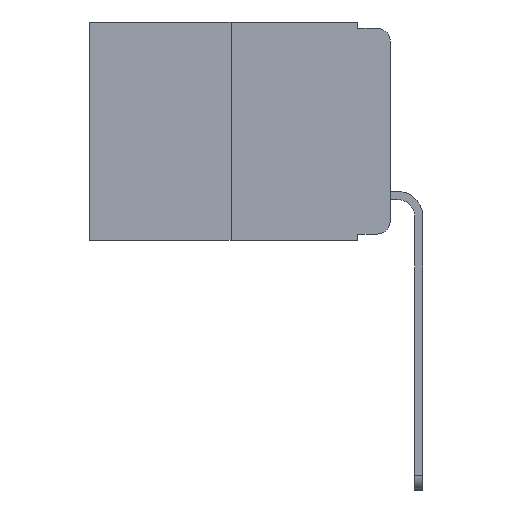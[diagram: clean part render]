
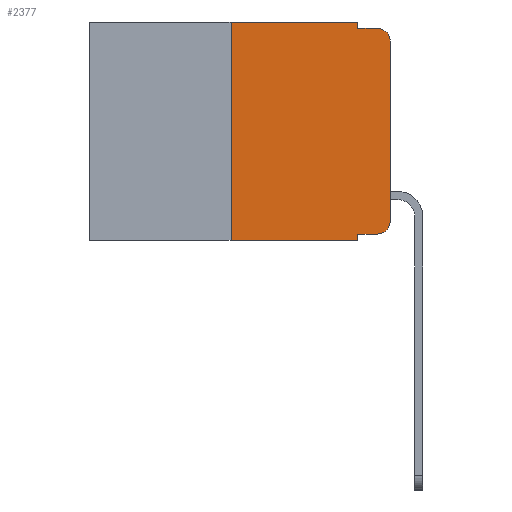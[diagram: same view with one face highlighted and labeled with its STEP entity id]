
A CAD part, left-side view. The second image highlights one B-rep face of the part: STEP entity #2377.
In plain terms, the highlighted planar face has unit normal (-1, 0, 0).
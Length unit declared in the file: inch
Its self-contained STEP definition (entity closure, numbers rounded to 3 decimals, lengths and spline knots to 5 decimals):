
#36 = VERTEX_POINT ( 'NONE', #1547 ) ;
#52 = DIRECTION ( 'NONE',  ( 0., 0., -1. ) ) ;
#395 = CARTESIAN_POINT ( 'NONE',  ( 0., 0.25, -0.343 ) ) ;
#418 = CARTESIAN_POINT ( 'NONE',  ( 0., 0.473, 0. ) ) ;
#467 = DIRECTION ( 'NONE',  ( 0., -1., 0. ) ) ;
#686 = EDGE_CURVE ( 'NONE', #36, #824, #2231, .T. ) ;
#691 = CARTESIAN_POINT ( 'NONE',  ( 0., 0.051, 0. ) ) ;
#729 = DIRECTION ( 'NONE',  ( 0., 0., -1. ) ) ;
#824 = VERTEX_POINT ( 'NONE', #7300 ) ;
#953 = VERTEX_POINT ( 'NONE', #4341 ) ;
#1054 = CARTESIAN_POINT ( 'NONE',  ( 0., 0.051, -0.343 ) ) ;
#1134 = FACE_OUTER_BOUND ( 'NONE', #9047, .T. ) ;
#1243 = PLANE ( 'NONE',  #7035 ) ;
#1254 = VERTEX_POINT ( 'NONE', #1486 ) ;
#1359 = DIRECTION ( 'NONE',  ( 0., -1., 0. ) ) ;
#1404 = VECTOR ( 'NONE', #2991, 39.37008 ) ;
#1415 = VECTOR ( 'NONE', #467, 39.37008 ) ;
#1481 = CARTESIAN_POINT ( 'NONE',  ( 0., 0.02, -0.03 ) ) ;
#1486 = CARTESIAN_POINT ( 'NONE',  ( 0., 0.25, 0. ) ) ;
#1547 = CARTESIAN_POINT ( 'NONE',  ( 0., 0., -0.313 ) ) ;
#1707 = LINE ( 'NONE', #6766, #1415 ) ;
#1807 = ORIENTED_EDGE ( 'NONE', *, *, #2525, .F. ) ;
#2095 = AXIS2_PLACEMENT_3D ( 'NONE', #10485, #5573, #52 ) ;
#2165 = LINE ( 'NONE', #691, #8855 ) ;
#2231 = LINE ( 'NONE', #6625, #8914 ) ;
#2274 = EDGE_CURVE ( 'NONE', #9213, #4367, #7803, .T. ) ;
#2282 = ORIENTED_EDGE ( 'NONE', *, *, #2274, .T. ) ;
#2377 = ADVANCED_FACE ( 'NONE', ( #1134 ), #1243, .F. ) ;
#2443 = VECTOR ( 'NONE', #3425, 39.37008 ) ;
#2459 = DIRECTION ( 'NONE',  ( 0., 0., -1. ) ) ;
#2525 = EDGE_CURVE ( 'NONE', #953, #3752, #8345, .T. ) ;
#2658 = DIRECTION ( 'NONE',  ( 1., 0., 0. ) ) ;
#2928 = VERTEX_POINT ( 'NONE', #1054 ) ;
#2991 = DIRECTION ( 'NONE',  ( 0., 0., 1. ) ) ;
#3024 = DIRECTION ( 'NONE',  ( 0., 0., -1. ) ) ;
#3425 = DIRECTION ( 'NONE',  ( 0., 0., -1. ) ) ;
#3752 = VERTEX_POINT ( 'NONE', #8951 ) ;
#3774 = VECTOR ( 'NONE', #8060, 39.37008 ) ;
#4341 = CARTESIAN_POINT ( 'NONE',  ( 0., 0.051, -0.01 ) ) ;
#4367 = VERTEX_POINT ( 'NONE', #6463 ) ;
#4823 = LINE ( 'NONE', #7467, #2443 ) ;
#4951 = ORIENTED_EDGE ( 'NONE', *, *, #10272, .F. ) ;
#5102 = CIRCLE ( 'NONE', #2095, 0.02 ) ;
#5226 = EDGE_CURVE ( 'NONE', #1254, #7766, #9955, .T. ) ;
#5386 = ORIENTED_EDGE ( 'NONE', *, *, #9959, .F. ) ;
#5524 = CARTESIAN_POINT ( 'NONE',  ( 0., 0.051, -0.333 ) ) ;
#5573 = DIRECTION ( 'NONE',  ( -1., 0., 0. ) ) ;
#5661 = ORIENTED_EDGE ( 'NONE', *, *, #6136, .F. ) ;
#5912 = DIRECTION ( 'NONE',  ( 0., 0., 1. ) ) ;
#6136 = EDGE_CURVE ( 'NONE', #7766, #953, #4823, .T. ) ;
#6405 = VECTOR ( 'NONE', #1359, 39.37008 ) ;
#6436 = CARTESIAN_POINT ( 'NONE',  ( 0., 0.051, 0. ) ) ;
#6463 = CARTESIAN_POINT ( 'NONE',  ( 0., 0.02, -0.333 ) ) ;
#6625 = CARTESIAN_POINT ( 'NONE',  ( 0., 0., 0. ) ) ;
#6766 = CARTESIAN_POINT ( 'NONE',  ( 0., 0.473, -0.343 ) ) ;
#7035 = AXIS2_PLACEMENT_3D ( 'NONE', #418, #2658, #3024 ) ;
#7077 = CARTESIAN_POINT ( 'NONE',  ( 0., 0.051, -0.333 ) ) ;
#7300 = CARTESIAN_POINT ( 'NONE',  ( 0., 0., -0.03 ) ) ;
#7354 = EDGE_CURVE ( 'NONE', #824, #3752, #10633, .T. ) ;
#7467 = CARTESIAN_POINT ( 'NONE',  ( 0., 0.051, 0. ) ) ;
#7542 = VECTOR ( 'NONE', #8374, 39.37008 ) ;
#7674 = DIRECTION ( 'NONE',  ( -1., 0., 0. ) ) ;
#7766 = VERTEX_POINT ( 'NONE', #6436 ) ;
#7803 = LINE ( 'NONE', #5524, #7542 ) ;
#8002 = ORIENTED_EDGE ( 'NONE', *, *, #686, .T. ) ;
#8012 = CARTESIAN_POINT ( 'NONE',  ( 0., 0.473, 0. ) ) ;
#8060 = DIRECTION ( 'NONE',  ( 0., -1., 0. ) ) ;
#8151 = ORIENTED_EDGE ( 'NONE', *, *, #5226, .F. ) ;
#8159 = CARTESIAN_POINT ( 'NONE',  ( 0., 0.25, 0. ) ) ;
#8287 = ORIENTED_EDGE ( 'NONE', *, *, #7354, .T. ) ;
#8345 = LINE ( 'NONE', #10754, #6405 ) ;
#8374 = DIRECTION ( 'NONE',  ( 0., -1., 0. ) ) ;
#8824 = VERTEX_POINT ( 'NONE', #395 ) ;
#8855 = VECTOR ( 'NONE', #729, 39.37008 ) ;
#8914 = VECTOR ( 'NONE', #5912, 39.37008 ) ;
#8951 = CARTESIAN_POINT ( 'NONE',  ( 0., 0.02, -0.01 ) ) ;
#9047 = EDGE_LOOP ( 'NONE', ( #8002, #8287, #1807, #5661, #8151, #4951, #9679, #5386, #2282, #10711 ) ) ;
#9213 = VERTEX_POINT ( 'NONE', #7077 ) ;
#9525 = AXIS2_PLACEMENT_3D ( 'NONE', #1481, #7674, #2459 ) ;
#9679 = ORIENTED_EDGE ( 'NONE', *, *, #9746, .T. ) ;
#9746 = EDGE_CURVE ( 'NONE', #8824, #2928, #1707, .T. ) ;
#9955 = LINE ( 'NONE', #8012, #3774 ) ;
#9959 = EDGE_CURVE ( 'NONE', #9213, #2928, #2165, .T. ) ;
#10272 = EDGE_CURVE ( 'NONE', #8824, #1254, #10554, .T. ) ;
#10485 = CARTESIAN_POINT ( 'NONE',  ( 0., 0.02, -0.313 ) ) ;
#10554 = LINE ( 'NONE', #8159, #1404 ) ;
#10633 = CIRCLE ( 'NONE', #9525, 0.02 ) ;
#10711 = ORIENTED_EDGE ( 'NONE', *, *, #10972, .T. ) ;
#10754 = CARTESIAN_POINT ( 'NONE',  ( 0., 0.051, -0.01 ) ) ;
#10972 = EDGE_CURVE ( 'NONE', #4367, #36, #5102, .T. ) ;
